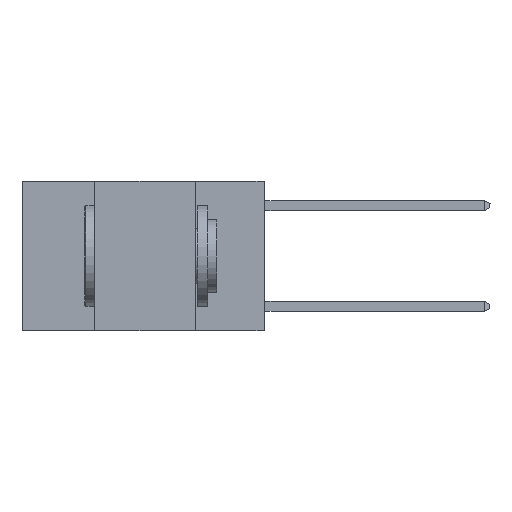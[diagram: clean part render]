
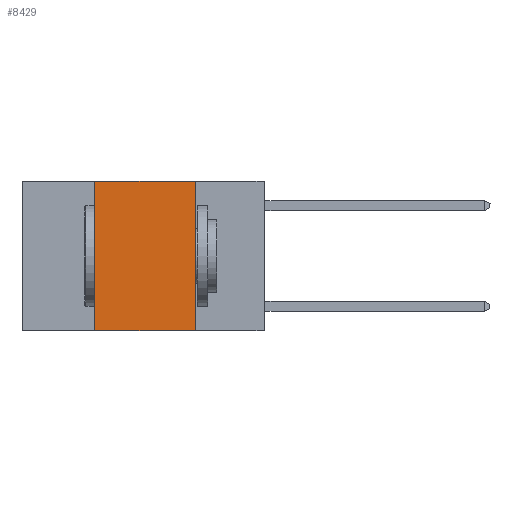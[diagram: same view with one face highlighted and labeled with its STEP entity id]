
A CAD part, left-side view. The second image highlights one B-rep face of the part: STEP entity #8429.
In plain terms, the highlighted planar face has unit normal (-1, 0, 0).
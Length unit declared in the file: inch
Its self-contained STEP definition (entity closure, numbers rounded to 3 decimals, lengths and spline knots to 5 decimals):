
#132 = VECTOR ( 'NONE', #17181, 39.37008 ) ;
#447 = EDGE_CURVE ( 'NONE', #12967, #14770, #1499, .T. ) ;
#1499 = LINE ( 'NONE', #19316, #15217 ) ;
#2592 = AXIS2_PLACEMENT_3D ( 'NONE', #8848, #17114, #9660 ) ;
#2882 = PLANE ( 'NONE',  #2592 ) ;
#3319 = VERTEX_POINT ( 'NONE', #12718 ) ;
#3991 = CARTESIAN_POINT ( 'NONE',  ( 0., 0.6, 0. ) ) ;
#5058 = LINE ( 'NONE', #15256, #13897 ) ;
#5553 = EDGE_CURVE ( 'NONE', #3319, #9909, #11100, .T. ) ;
#6017 = VECTOR ( 'NONE', #18695, 39.37008 ) ;
#6225 = ORIENTED_EDGE ( 'NONE', *, *, #7875, .F. ) ;
#7430 = CARTESIAN_POINT ( 'NONE',  ( 0., 0.42, -0.37 ) ) ;
#7536 = CARTESIAN_POINT ( 'NONE',  ( 0., 0.17, -0.37 ) ) ;
#7875 = EDGE_CURVE ( 'NONE', #14770, #3319, #9893, .T. ) ;
#8429 = ADVANCED_FACE ( 'NONE', ( #10333 ), #2882, .F. ) ;
#8848 = CARTESIAN_POINT ( 'NONE',  ( 0., 0.6, 0. ) ) ;
#8972 = ORIENTED_EDGE ( 'NONE', *, *, #5553, .F. ) ;
#9660 = DIRECTION ( 'NONE',  ( 0., 0., -1. ) ) ;
#9893 = LINE ( 'NONE', #3991, #6017 ) ;
#9909 = VERTEX_POINT ( 'NONE', #7536 ) ;
#10333 = FACE_OUTER_BOUND ( 'NONE', #10752, .T. ) ;
#10752 = EDGE_LOOP ( 'NONE', ( #8972, #6225, #15390, #13997 ) ) ;
#11100 = LINE ( 'NONE', #18263, #132 ) ;
#12718 = CARTESIAN_POINT ( 'NONE',  ( 0., 0.17, 0. ) ) ;
#12967 = VERTEX_POINT ( 'NONE', #7430 ) ;
#13897 = VECTOR ( 'NONE', #18300, 39.37008 ) ;
#13997 = ORIENTED_EDGE ( 'NONE', *, *, #19195, .T. ) ;
#14770 = VERTEX_POINT ( 'NONE', #18922 ) ;
#15111 = DIRECTION ( 'NONE',  ( 0., 0., 1. ) ) ;
#15217 = VECTOR ( 'NONE', #15111, 39.37008 ) ;
#15256 = CARTESIAN_POINT ( 'NONE',  ( 0., 0.6, -0.37 ) ) ;
#15390 = ORIENTED_EDGE ( 'NONE', *, *, #447, .F. ) ;
#17114 = DIRECTION ( 'NONE',  ( 1., 0., 0. ) ) ;
#17181 = DIRECTION ( 'NONE',  ( 0., 0., -1. ) ) ;
#18263 = CARTESIAN_POINT ( 'NONE',  ( 0., 0.17, 0. ) ) ;
#18300 = DIRECTION ( 'NONE',  ( 0., -1., 0. ) ) ;
#18695 = DIRECTION ( 'NONE',  ( 0., -1., 0. ) ) ;
#18922 = CARTESIAN_POINT ( 'NONE',  ( 0., 0.42, 0. ) ) ;
#19195 = EDGE_CURVE ( 'NONE', #12967, #9909, #5058, .T. ) ;
#19316 = CARTESIAN_POINT ( 'NONE',  ( 0., 0.42, 0. ) ) ;
